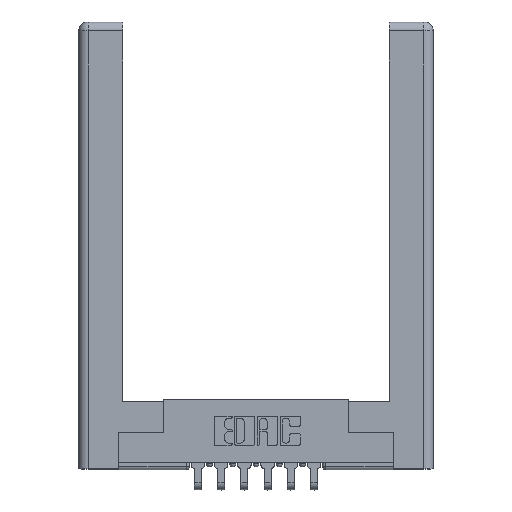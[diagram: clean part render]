
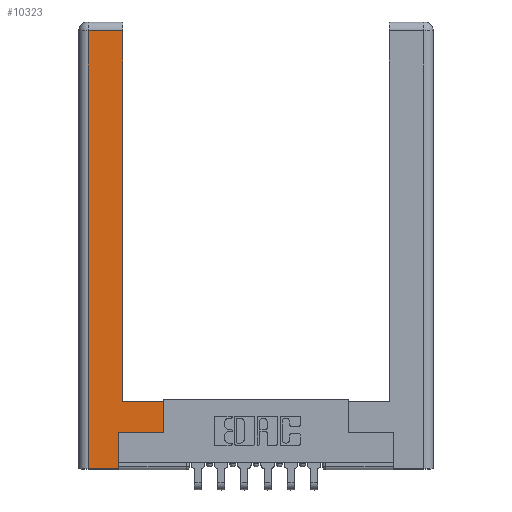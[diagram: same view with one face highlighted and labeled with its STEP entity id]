
A CAD part, top view. The second image highlights one B-rep face of the part: STEP entity #10323.
In plain terms, the highlighted planar face has unit normal (0, 0, 1).
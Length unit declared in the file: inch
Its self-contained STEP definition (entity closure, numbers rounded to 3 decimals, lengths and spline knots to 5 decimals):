
#57 = EDGE_CURVE ( 'NONE', #4910, #527, #154, .T. ) ;
#144 = VECTOR ( 'NONE', #5509, 39.37008 ) ;
#154 = LINE ( 'NONE', #4600, #4902 ) ;
#288 = ORIENTED_EDGE ( 'NONE', *, *, #12053, .T. ) ;
#527 = VERTEX_POINT ( 'NONE', #9992 ) ;
#859 = VERTEX_POINT ( 'NONE', #4488 ) ;
#936 = DIRECTION ( 'NONE',  ( 1., 0., 0. ) ) ;
#956 = ORIENTED_EDGE ( 'NONE', *, *, #11787, .T. ) ;
#1210 = DIRECTION ( 'NONE',  ( 1., 0., 0. ) ) ;
#1304 = DIRECTION ( 'NONE',  ( 0., 1., 0. ) ) ;
#1377 = PLANE ( 'NONE',  #9387 ) ;
#1592 = LINE ( 'NONE', #3344, #11414 ) ;
#1669 = VERTEX_POINT ( 'NONE', #11339 ) ;
#1683 = CARTESIAN_POINT ( 'NONE',  ( 0.0615, 2.94, 0. ) ) ;
#2092 = CARTESIAN_POINT ( 'NONE',  ( 0.0615, 0., 0. ) ) ;
#2279 = CARTESIAN_POINT ( 'NONE',  ( 0.565, 0.45, 0. ) ) ;
#2291 = VECTOR ( 'NONE', #3276, 39.37008 ) ;
#2396 = ORIENTED_EDGE ( 'NONE', *, *, #57, .T. ) ;
#2457 = ORIENTED_EDGE ( 'NONE', *, *, #4462, .T. ) ;
#2494 = CARTESIAN_POINT ( 'NONE',  ( 0., 0., 0. ) ) ;
#2554 = CARTESIAN_POINT ( 'NONE',  ( 0.295, 0.45, 0. ) ) ;
#2644 = CARTESIAN_POINT ( 'NONE',  ( 0.565, 0.245, 0. ) ) ;
#2679 = DIRECTION ( 'NONE',  ( -1., 0., 0. ) ) ;
#2905 = VECTOR ( 'NONE', #1210, 39.37008 ) ;
#3100 = ORIENTED_EDGE ( 'NONE', *, *, #6111, .T. ) ;
#3276 = DIRECTION ( 'NONE',  ( 0., 1., 0. ) ) ;
#3338 = LINE ( 'NONE', #3875, #12156 ) ;
#3344 = CARTESIAN_POINT ( 'NONE',  ( 0.0615, 0., 0. ) ) ;
#3508 = VECTOR ( 'NONE', #2679, 39.37008 ) ;
#3544 = EDGE_LOOP ( 'NONE', ( #2396, #5384, #10619, #2457, #288, #956, #6285, #3100 ) ) ;
#3870 = EDGE_CURVE ( 'NONE', #11231, #1669, #4533, .T. ) ;
#3875 = CARTESIAN_POINT ( 'NONE',  ( 0.565, 0.245, 0. ) ) ;
#4446 = LINE ( 'NONE', #2554, #144 ) ;
#4462 = EDGE_CURVE ( 'NONE', #10120, #5120, #6969, .T. ) ;
#4488 = CARTESIAN_POINT ( 'NONE',  ( 0.265, 0.245, 0. ) ) ;
#4533 = LINE ( 'NONE', #2279, #2291 ) ;
#4600 = CARTESIAN_POINT ( 'NONE',  ( 0.295, 3., 0. ) ) ;
#4902 = VECTOR ( 'NONE', #11251, 39.37008 ) ;
#4910 = VERTEX_POINT ( 'NONE', #6448 ) ;
#5120 = VERTEX_POINT ( 'NONE', #5493 ) ;
#5127 = LINE ( 'NONE', #7023, #7361 ) ;
#5384 = ORIENTED_EDGE ( 'NONE', *, *, #11149, .T. ) ;
#5493 = CARTESIAN_POINT ( 'NONE',  ( 0.265, 0., 0. ) ) ;
#5509 = DIRECTION ( 'NONE',  ( -1., 0., 0. ) ) ;
#5930 = CARTESIAN_POINT ( 'NONE',  ( 0.265, 0., 0. ) ) ;
#6111 = EDGE_CURVE ( 'NONE', #1669, #4910, #4446, .T. ) ;
#6171 = DIRECTION ( 'NONE',  ( 0., -1., 0. ) ) ;
#6285 = ORIENTED_EDGE ( 'NONE', *, *, #3870, .T. ) ;
#6332 = LINE ( 'NONE', #1683, #3508 ) ;
#6448 = CARTESIAN_POINT ( 'NONE',  ( 0.295, 0.45, 0. ) ) ;
#6969 = LINE ( 'NONE', #5930, #2905 ) ;
#6997 = EDGE_CURVE ( 'NONE', #11031, #10120, #1592, .T. ) ;
#7023 = CARTESIAN_POINT ( 'NONE',  ( 0.265, 0.245, 0. ) ) ;
#7301 = CARTESIAN_POINT ( 'NONE',  ( 0.0615, 2.94, 0. ) ) ;
#7361 = VECTOR ( 'NONE', #1304, 39.37008 ) ;
#8044 = FACE_OUTER_BOUND ( 'NONE', #3544, .T. ) ;
#9387 = AXIS2_PLACEMENT_3D ( 'NONE', #2494, #11944, #10089 ) ;
#9992 = CARTESIAN_POINT ( 'NONE',  ( 0.295, 2.94, 0. ) ) ;
#10089 = DIRECTION ( 'NONE',  ( -1., 0., 0. ) ) ;
#10120 = VERTEX_POINT ( 'NONE', #2092 ) ;
#10323 = ADVANCED_FACE ( 'NONE', ( #8044 ), #1377, .F. ) ;
#10619 = ORIENTED_EDGE ( 'NONE', *, *, #6997, .T. ) ;
#11031 = VERTEX_POINT ( 'NONE', #7301 ) ;
#11149 = EDGE_CURVE ( 'NONE', #527, #11031, #6332, .T. ) ;
#11231 = VERTEX_POINT ( 'NONE', #2644 ) ;
#11251 = DIRECTION ( 'NONE',  ( 0., 1., 0. ) ) ;
#11339 = CARTESIAN_POINT ( 'NONE',  ( 0.565, 0.45, 0. ) ) ;
#11414 = VECTOR ( 'NONE', #6171, 39.37008 ) ;
#11787 = EDGE_CURVE ( 'NONE', #859, #11231, #3338, .T. ) ;
#11944 = DIRECTION ( 'NONE',  ( 0., 0., -1. ) ) ;
#12053 = EDGE_CURVE ( 'NONE', #5120, #859, #5127, .T. ) ;
#12156 = VECTOR ( 'NONE', #936, 39.37008 ) ;
